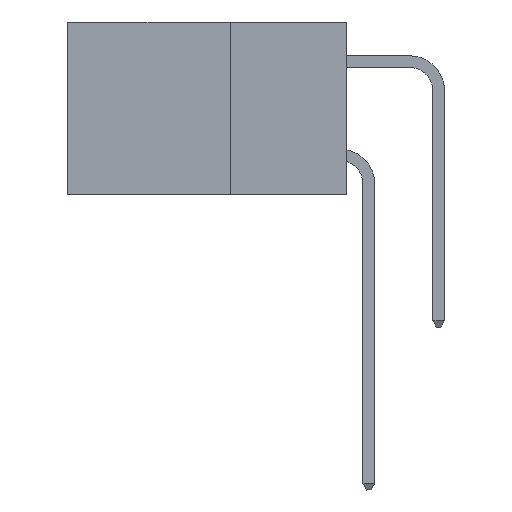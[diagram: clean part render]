
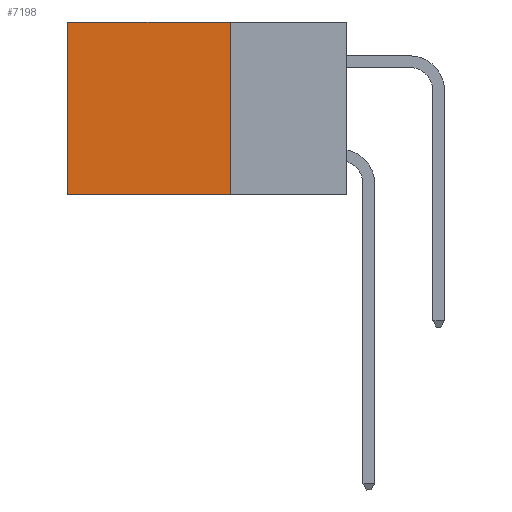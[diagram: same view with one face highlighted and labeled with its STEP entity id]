
A CAD part, left-side view. The second image highlights one B-rep face of the part: STEP entity #7198.
In plain terms, the highlighted planar face has unit normal (-1, 0, 0).
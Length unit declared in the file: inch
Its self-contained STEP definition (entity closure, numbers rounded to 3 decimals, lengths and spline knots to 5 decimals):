
#1510 = LINE ( 'NONE', #20689, #6201 ) ;
#1952 = DIRECTION ( 'NONE',  ( 1., 0., 0. ) ) ;
#2068 = DIRECTION ( 'NONE',  ( 0., 1., 0. ) ) ;
#3842 = DIRECTION ( 'NONE',  ( 0., 1., 0. ) ) ;
#4304 = LINE ( 'NONE', #20533, #8961 ) ;
#5882 = VECTOR ( 'NONE', #2068, 39.37008 ) ;
#6140 = ORIENTED_EDGE ( 'NONE', *, *, #20261, .F. ) ;
#6201 = VECTOR ( 'NONE', #18770, 39.37008 ) ;
#6479 = LINE ( 'NONE', #12015, #5882 ) ;
#6787 = AXIS2_PLACEMENT_3D ( 'NONE', #9876, #1952, #15789 ) ;
#7198 = ADVANCED_FACE ( 'NONE', ( #9980 ), #13865, .F. ) ;
#7729 = VECTOR ( 'NONE', #3842, 39.37008 ) ;
#8076 = VERTEX_POINT ( 'NONE', #12545 ) ;
#8246 = EDGE_CURVE ( 'NONE', #21773, #11940, #1510, .T. ) ;
#8961 = VECTOR ( 'NONE', #22467, 39.37008 ) ;
#9876 = CARTESIAN_POINT ( 'NONE',  ( 0.2875, 0.25, 0. ) ) ;
#9980 = FACE_OUTER_BOUND ( 'NONE', #18195, .T. ) ;
#10639 = CARTESIAN_POINT ( 'NONE',  ( 0.2875, 0.6, 0. ) ) ;
#11940 = VERTEX_POINT ( 'NONE', #16043 ) ;
#12015 = CARTESIAN_POINT ( 'NONE',  ( 0.2875, 0.25, 0. ) ) ;
#12273 = ORIENTED_EDGE ( 'NONE', *, *, #19944, .F. ) ;
#12545 = CARTESIAN_POINT ( 'NONE',  ( 0.2875, 0.25, -0.37 ) ) ;
#13865 = PLANE ( 'NONE',  #6787 ) ;
#15789 = DIRECTION ( 'NONE',  ( 0., 0., -1. ) ) ;
#16012 = CARTESIAN_POINT ( 'NONE',  ( 0.2875, 0.25, 0. ) ) ;
#16043 = CARTESIAN_POINT ( 'NONE',  ( 0.2875, 0.6, -0.37 ) ) ;
#17590 = CARTESIAN_POINT ( 'NONE',  ( 0.2875, 0.25, -0.37 ) ) ;
#18195 = EDGE_LOOP ( 'NONE', ( #21853, #6140, #12273, #21672 ) ) ;
#18748 = LINE ( 'NONE', #17590, #7729 ) ;
#18770 = DIRECTION ( 'NONE',  ( 0., 0., -1. ) ) ;
#19944 = EDGE_CURVE ( 'NONE', #23659, #8076, #4304, .T. ) ;
#20261 = EDGE_CURVE ( 'NONE', #8076, #11940, #18748, .T. ) ;
#20312 = EDGE_CURVE ( 'NONE', #23659, #21773, #6479, .T. ) ;
#20533 = CARTESIAN_POINT ( 'NONE',  ( 0.2875, 0.25, 0. ) ) ;
#20689 = CARTESIAN_POINT ( 'NONE',  ( 0.2875, 0.6, 0. ) ) ;
#21672 = ORIENTED_EDGE ( 'NONE', *, *, #20312, .T. ) ;
#21773 = VERTEX_POINT ( 'NONE', #10639 ) ;
#21853 = ORIENTED_EDGE ( 'NONE', *, *, #8246, .T. ) ;
#22467 = DIRECTION ( 'NONE',  ( 0., 0., -1. ) ) ;
#23659 = VERTEX_POINT ( 'NONE', #16012 ) ;
